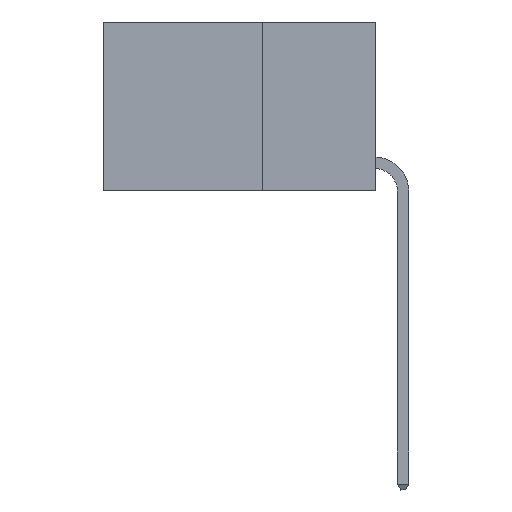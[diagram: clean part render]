
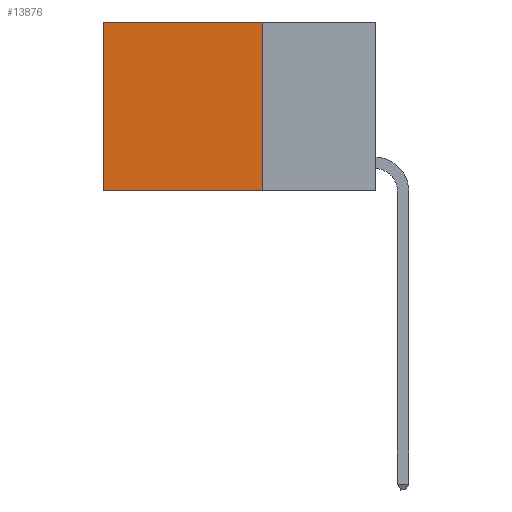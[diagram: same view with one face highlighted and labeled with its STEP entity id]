
A CAD part, left-side view. The second image highlights one B-rep face of the part: STEP entity #13876.
In plain terms, the highlighted planar face has unit normal (-1, 0, 0).
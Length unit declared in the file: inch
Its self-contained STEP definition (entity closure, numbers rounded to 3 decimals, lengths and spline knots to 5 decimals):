
#690 = DIRECTION ( 'NONE',  ( 0., 0., -1. ) ) ;
#798 = ORIENTED_EDGE ( 'NONE', *, *, #14081, .F. ) ;
#1442 = VECTOR ( 'NONE', #13657, 39.37008 ) ;
#2227 = CARTESIAN_POINT ( 'NONE',  ( 0.2625, 0.25, -0.37 ) ) ;
#2279 = CARTESIAN_POINT ( 'NONE',  ( 0.2625, 0.6, 0. ) ) ;
#2954 = DIRECTION ( 'NONE',  ( 1., 0., 0. ) ) ;
#4729 = LINE ( 'NONE', #2227, #4817 ) ;
#4817 = VECTOR ( 'NONE', #11567, 39.37008 ) ;
#5186 = CARTESIAN_POINT ( 'NONE',  ( 0.2625, 0.25, 0. ) ) ;
#5325 = ORIENTED_EDGE ( 'NONE', *, *, #7784, .T. ) ;
#5514 = EDGE_CURVE ( 'NONE', #14566, #12125, #11243, .T. ) ;
#5856 = LINE ( 'NONE', #10486, #14779 ) ;
#5915 = VECTOR ( 'NONE', #10664, 39.37008 ) ;
#6025 = LINE ( 'NONE', #6098, #5915 ) ;
#6098 = CARTESIAN_POINT ( 'NONE',  ( 0.2625, 0.25, 0. ) ) ;
#6391 = VERTEX_POINT ( 'NONE', #13622 ) ;
#6498 = CARTESIAN_POINT ( 'NONE',  ( 0.2625, 0.6, -0.37 ) ) ;
#6665 = VERTEX_POINT ( 'NONE', #5186 ) ;
#7035 = EDGE_CURVE ( 'NONE', #6391, #12125, #4729, .T. ) ;
#7574 = CARTESIAN_POINT ( 'NONE',  ( 0.2625, 0.6, 0. ) ) ;
#7784 = EDGE_CURVE ( 'NONE', #6665, #14566, #5856, .T. ) ;
#7909 = ORIENTED_EDGE ( 'NONE', *, *, #5514, .T. ) ;
#8931 = ORIENTED_EDGE ( 'NONE', *, *, #7035, .F. ) ;
#9769 = CARTESIAN_POINT ( 'NONE',  ( 0.2625, 0.25, 0. ) ) ;
#10486 = CARTESIAN_POINT ( 'NONE',  ( 0.2625, 0.25, 0. ) ) ;
#10664 = DIRECTION ( 'NONE',  ( 0., 0., -1. ) ) ;
#10880 = EDGE_LOOP ( 'NONE', ( #7909, #8931, #798, #5325 ) ) ;
#11243 = LINE ( 'NONE', #2279, #1442 ) ;
#11567 = DIRECTION ( 'NONE',  ( 0., 1., 0. ) ) ;
#12125 = VERTEX_POINT ( 'NONE', #6498 ) ;
#12973 = DIRECTION ( 'NONE',  ( 0., 1., 0. ) ) ;
#13414 = FACE_OUTER_BOUND ( 'NONE', #10880, .T. ) ;
#13622 = CARTESIAN_POINT ( 'NONE',  ( 0.2625, 0.25, -0.37 ) ) ;
#13657 = DIRECTION ( 'NONE',  ( 0., 0., -1. ) ) ;
#13876 = ADVANCED_FACE ( 'NONE', ( #13414 ), #14477, .F. ) ;
#13904 = AXIS2_PLACEMENT_3D ( 'NONE', #9769, #2954, #690 ) ;
#14081 = EDGE_CURVE ( 'NONE', #6665, #6391, #6025, .T. ) ;
#14477 = PLANE ( 'NONE',  #13904 ) ;
#14566 = VERTEX_POINT ( 'NONE', #7574 ) ;
#14779 = VECTOR ( 'NONE', #12973, 39.37008 ) ;
